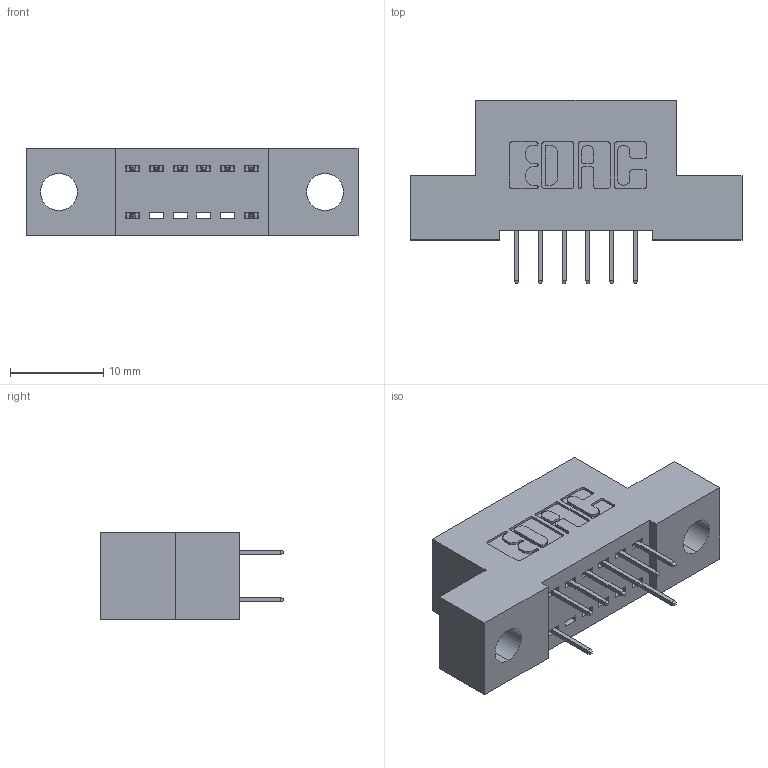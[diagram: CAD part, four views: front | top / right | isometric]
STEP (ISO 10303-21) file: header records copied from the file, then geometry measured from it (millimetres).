
FILE_DESCRIPTION (( 'STEP AP203' ), '1' );
FILE_NAME ('392-012-524-204.STEP', '2018-08-14T21:59:04', ( '' ), ( '' ), 'SwSTEP 2.0', 'SolidWorks 2016', '' );
FILE_SCHEMA (( 'CONFIG_CONTROL_DESIGN' ));
Length unit declared in the file: inch
Products named in the file (3): 345-292-001_345-293-124; 392-012-524-204; 342 Part_.156 TH
Assembly tree (9 placements, depth 2):
  392-012-524-204
    342 Part_.156 TH
    345-292-001_345-293-124  x8
Bounding box: 35.56 x 19.69 x 9.4 mm (x, y, z)
Volume: 2889.5 mm3; surface area: 3410.1 mm2
Topology: 9 solids, 9 shells, 582 faces, 1655 edges, 1070 vertices
Faces by surface type: plane 426, cylinder 156
Entity records: 8333 total; most frequent: CARTESIAN_POINT 1438, ORIENTED_EDGE 1378, DIRECTION 1289, EDGE_CURVE 689, VECTOR 565, LINE 565, VERTEX_POINT 454, AXIS2_PLACEMENT_3D 362
